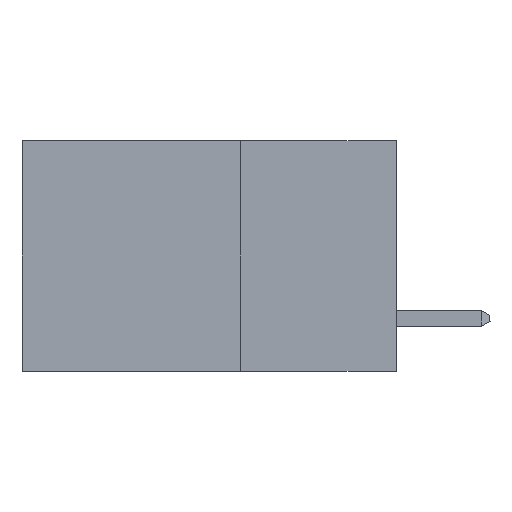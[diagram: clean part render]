
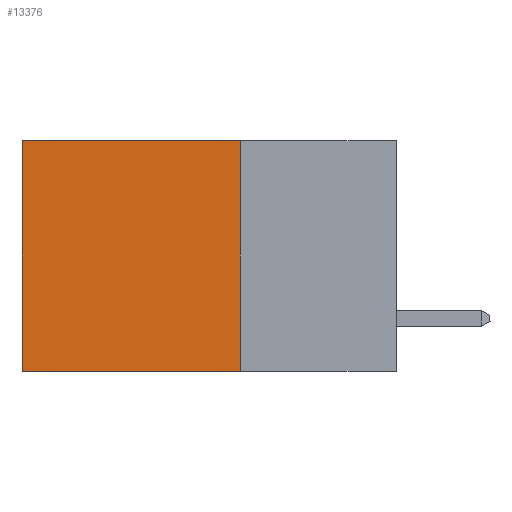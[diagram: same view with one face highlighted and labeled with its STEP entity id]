
A CAD part, left-side view. The second image highlights one B-rep face of the part: STEP entity #13376.
In plain terms, the highlighted planar face has unit normal (-1, 0, 0).
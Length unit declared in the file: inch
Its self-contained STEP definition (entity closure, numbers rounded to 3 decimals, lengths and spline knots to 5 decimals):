
#230 = CARTESIAN_POINT ( 'NONE',  ( 0.298, 0.25, 0. ) ) ;
#473 = VECTOR ( 'NONE', #2761, 39.37008 ) ;
#485 = EDGE_CURVE ( 'NONE', #12888, #3609, #5838, .T. ) ;
#628 = DIRECTION ( 'NONE',  ( 0., 0., -1. ) ) ;
#680 = PLANE ( 'NONE',  #15874 ) ;
#1435 = EDGE_LOOP ( 'NONE', ( #1824, #8729, #12989, #12919 ) ) ;
#1824 = ORIENTED_EDGE ( 'NONE', *, *, #5691, .T. ) ;
#2761 = DIRECTION ( 'NONE',  ( 0., 0., -1. ) ) ;
#2859 = CARTESIAN_POINT ( 'NONE',  ( 0.298, 0.25, -0.37 ) ) ;
#2974 = VECTOR ( 'NONE', #14587, 39.37008 ) ;
#3609 = VERTEX_POINT ( 'NONE', #5544 ) ;
#3799 = CARTESIAN_POINT ( 'NONE',  ( 0.298, 0.25, 0. ) ) ;
#4136 = VERTEX_POINT ( 'NONE', #9280 ) ;
#4391 = EDGE_CURVE ( 'NONE', #12888, #4136, #9532, .T. ) ;
#4629 = CARTESIAN_POINT ( 'NONE',  ( 0.298, 0.6, 0. ) ) ;
#5289 = DIRECTION ( 'NONE',  ( 0., 1., 0. ) ) ;
#5467 = DIRECTION ( 'NONE',  ( 0., 1., 0. ) ) ;
#5544 = CARTESIAN_POINT ( 'NONE',  ( 0.298, 0.25, -0.37 ) ) ;
#5691 = EDGE_CURVE ( 'NONE', #4136, #6379, #13126, .T. ) ;
#5838 = LINE ( 'NONE', #11646, #473 ) ;
#6379 = VERTEX_POINT ( 'NONE', #11067 ) ;
#7084 = EDGE_CURVE ( 'NONE', #3609, #6379, #13847, .T. ) ;
#7348 = FACE_OUTER_BOUND ( 'NONE', #1435, .T. ) ;
#8729 = ORIENTED_EDGE ( 'NONE', *, *, #7084, .F. ) ;
#9280 = CARTESIAN_POINT ( 'NONE',  ( 0.298, 0.6, 0. ) ) ;
#9450 = CARTESIAN_POINT ( 'NONE',  ( 0.298, 0.25, 0. ) ) ;
#9532 = LINE ( 'NONE', #230, #9907 ) ;
#9907 = VECTOR ( 'NONE', #5289, 39.37008 ) ;
#11067 = CARTESIAN_POINT ( 'NONE',  ( 0.298, 0.6, -0.37 ) ) ;
#11646 = CARTESIAN_POINT ( 'NONE',  ( 0.298, 0.25, 0. ) ) ;
#12447 = VECTOR ( 'NONE', #5467, 39.37008 ) ;
#12888 = VERTEX_POINT ( 'NONE', #3799 ) ;
#12919 = ORIENTED_EDGE ( 'NONE', *, *, #4391, .T. ) ;
#12989 = ORIENTED_EDGE ( 'NONE', *, *, #485, .F. ) ;
#13126 = LINE ( 'NONE', #4629, #2974 ) ;
#13376 = ADVANCED_FACE ( 'NONE', ( #7348 ), #680, .F. ) ;
#13847 = LINE ( 'NONE', #2859, #12447 ) ;
#14587 = DIRECTION ( 'NONE',  ( 0., 0., -1. ) ) ;
#15874 = AXIS2_PLACEMENT_3D ( 'NONE', #9450, #16010, #628 ) ;
#16010 = DIRECTION ( 'NONE',  ( 1., 0., 0. ) ) ;
